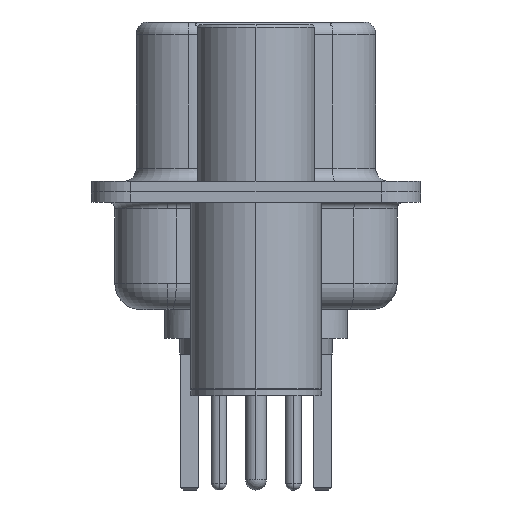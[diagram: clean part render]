
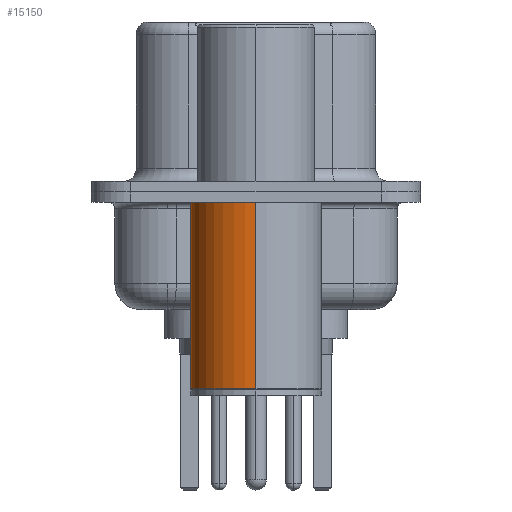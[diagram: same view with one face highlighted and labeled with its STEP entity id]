
A CAD part, left-side view. The second image highlights one B-rep face of the part: STEP entity #15150.
In plain terms, the highlighted cylindrical face has radius 2.5 mm (diameter 5 mm), a partial arc.
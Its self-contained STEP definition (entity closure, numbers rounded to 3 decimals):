
#894 = EDGE_CURVE ( 'NONE', #19417, #3744, #1684, .T. ) ;
#1039 = EDGE_CURVE ( 'NONE', #19778, #8972, #23142, .T. ) ;
#1684 = CIRCLE ( 'NONE', #12810, 2.5 ) ;
#1832 = DIRECTION ( 'NONE',  ( 1., 0., 0. ) ) ;
#2053 = DIRECTION ( 'NONE',  ( 1., 0., 0. ) ) ;
#3506 = DIRECTION ( 'NONE',  ( 0., 0., 1. ) ) ;
#3691 = ORIENTED_EDGE ( 'NONE', *, *, #894, .F. ) ;
#3744 = VERTEX_POINT ( 'NONE', #21736 ) ;
#4152 = DIRECTION ( 'NONE',  ( 0., 0., 1. ) ) ;
#5484 = CARTESIAN_POINT ( 'NONE',  ( 0., 0., -0.4 ) ) ;
#5571 = CARTESIAN_POINT ( 'NONE',  ( -2.5, 0., 0.581 ) ) ;
#5928 = CARTESIAN_POINT ( 'NONE',  ( -2.5, 0., -7.525 ) ) ;
#6322 = ORIENTED_EDGE ( 'NONE', *, *, #7157, .T. ) ;
#7157 = EDGE_CURVE ( 'NONE', #8972, #3744, #21502, .T. ) ;
#8972 = VERTEX_POINT ( 'NONE', #5928 ) ;
#9087 = CARTESIAN_POINT ( 'NONE',  ( 0., 0., 0.581 ) ) ;
#9101 = LINE ( 'NONE', #11528, #19390 ) ;
#9502 = DIRECTION ( 'NONE',  ( 1., 0., 0. ) ) ;
#10507 = CARTESIAN_POINT ( 'NONE',  ( 2.5, 0., -0.4 ) ) ;
#11128 = DIRECTION ( 'NONE',  ( 0., 0., 1. ) ) ;
#11528 = CARTESIAN_POINT ( 'NONE',  ( 2.5, 0., 0.581 ) ) ;
#11583 = DIRECTION ( 'NONE',  ( 0., 0., 1. ) ) ;
#11704 = ORIENTED_EDGE ( 'NONE', *, *, #1039, .T. ) ;
#11749 = AXIS2_PLACEMENT_3D ( 'NONE', #9087, #12760, #1832 ) ;
#11752 = VECTOR ( 'NONE', #11128, 1000. ) ;
#11980 = EDGE_LOOP ( 'NONE', ( #11704, #6322, #3691, #22083 ) ) ;
#12358 = AXIS2_PLACEMENT_3D ( 'NONE', #16638, #11583, #9502 ) ;
#12462 = CYLINDRICAL_SURFACE ( 'NONE', #11749, 2.5 ) ;
#12760 = DIRECTION ( 'NONE',  ( 0., 0., 1. ) ) ;
#12810 = AXIS2_PLACEMENT_3D ( 'NONE', #5484, #3506, #2053 ) ;
#15150 = ADVANCED_FACE ( 'NONE', ( #17284 ), #12462, .T. ) ;
#16638 = CARTESIAN_POINT ( 'NONE',  ( 0., 0., -7.525 ) ) ;
#16647 = EDGE_CURVE ( 'NONE', #19778, #19417, #9101, .T. ) ;
#17284 = FACE_OUTER_BOUND ( 'NONE', #11980, .T. ) ;
#19390 = VECTOR ( 'NONE', #4152, 1000. ) ;
#19417 = VERTEX_POINT ( 'NONE', #10507 ) ;
#19778 = VERTEX_POINT ( 'NONE', #22510 ) ;
#21502 = LINE ( 'NONE', #5571, #11752 ) ;
#21736 = CARTESIAN_POINT ( 'NONE',  ( -2.5, 0., -0.4 ) ) ;
#22083 = ORIENTED_EDGE ( 'NONE', *, *, #16647, .F. ) ;
#22510 = CARTESIAN_POINT ( 'NONE',  ( 2.5, 0., -7.525 ) ) ;
#23142 = CIRCLE ( 'NONE', #12358, 2.5 ) ;
